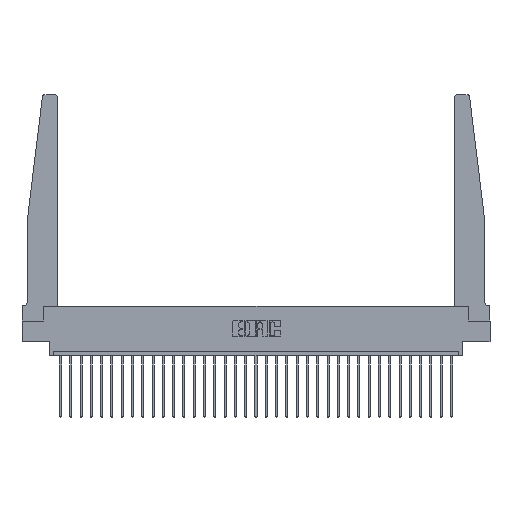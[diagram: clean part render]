
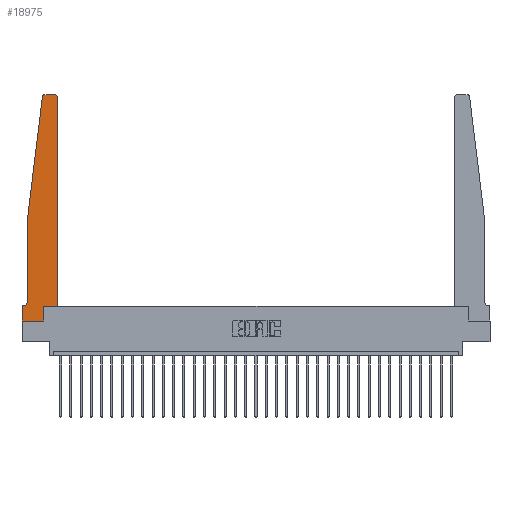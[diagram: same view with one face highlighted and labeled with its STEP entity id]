
A CAD part, top view. The second image highlights one B-rep face of the part: STEP entity #18975.
In plain terms, the highlighted planar face has unit normal (0, 0, 1).
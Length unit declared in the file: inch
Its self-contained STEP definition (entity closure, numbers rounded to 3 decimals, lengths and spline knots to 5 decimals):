
#232 = CARTESIAN_POINT ( 'NONE',  ( 0.065, 1.25, 0.37 ) ) ;
#612 = CARTESIAN_POINT ( 'NONE',  ( 0., 0.1875, 0.37 ) ) ;
#1583 = VERTEX_POINT ( 'NONE', #20414 ) ;
#1727 = DIRECTION ( 'NONE',  ( -1., 0., 0. ) ) ;
#2934 = VERTEX_POINT ( 'NONE', #27861 ) ;
#2939 = CARTESIAN_POINT ( 'NONE',  ( 0.27653, 2.72, 0.37 ) ) ;
#3016 = CARTESIAN_POINT ( 'NONE',  ( 0.065, 1.25, 0.37 ) ) ;
#3254 = AXIS2_PLACEMENT_3D ( 'NONE', #21858, #15500, #8918 ) ;
#3406 = VERTEX_POINT ( 'NONE', #26268 ) ;
#3511 = CARTESIAN_POINT ( 'NONE',  ( 0.395, 2.72, 0.37 ) ) ;
#3538 = CARTESIAN_POINT ( 'NONE',  ( 0.065, 1.25, 0.37 ) ) ;
#3747 = CARTESIAN_POINT ( 'NONE',  ( 0.065, 0.1875, 0.37 ) ) ;
#4135 = DIRECTION ( 'NONE',  ( 0., 0., -1. ) ) ;
#4173 = EDGE_CURVE ( 'NONE', #13566, #26030, #20560, .T. ) ;
#4426 = DIRECTION ( 'NONE',  ( 1., 0., 0. ) ) ;
#5262 = DIRECTION ( 'NONE',  ( 0., 1., 0. ) ) ;
#5278 = VERTEX_POINT ( 'NONE', #26256 ) ;
#5492 = CIRCLE ( 'NONE', #21734, 0.03 ) ;
#5751 = EDGE_CURVE ( 'NONE', #7166, #2934, #5492, .T. ) ;
#5842 = ORIENTED_EDGE ( 'NONE', *, *, #21548, .T. ) ;
#6036 = VERTEX_POINT ( 'NONE', #3538 ) ;
#6466 = CARTESIAN_POINT ( 'NONE',  ( 0.2605, 0.18, 0.37 ) ) ;
#6609 = ORIENTED_EDGE ( 'NONE', *, *, #5751, .T. ) ;
#6763 = EDGE_CURVE ( 'NONE', #5278, #23042, #8334, .T. ) ;
#7166 = VERTEX_POINT ( 'NONE', #9175 ) ;
#7581 = LINE ( 'NONE', #3747, #11492 ) ;
#7905 = CARTESIAN_POINT ( 'NONE',  ( 0.2605, 0., 0.37 ) ) ;
#8334 = CIRCLE ( 'NONE', #17591, 0.03 ) ;
#8335 = VECTOR ( 'NONE', #13988, 39.37008 ) ;
#8407 = EDGE_LOOP ( 'NONE', ( #16401, #24054, #27686, #21532, #26151, #25144, #13466, #16204, #27030, #24911, #5842, #6609 ) ) ;
#8863 = CARTESIAN_POINT ( 'NONE',  ( 0.24675, 2.72367, 0.37 ) ) ;
#8918 = DIRECTION ( 'NONE',  ( 1., 0., 0. ) ) ;
#9175 = CARTESIAN_POINT ( 'NONE',  ( 0.425, 2.72, 0.37 ) ) ;
#9806 = LINE ( 'NONE', #22741, #27277 ) ;
#9874 = DIRECTION ( 'NONE',  ( 0., 0., 1. ) ) ;
#10101 = LINE ( 'NONE', #3016, #8335 ) ;
#10420 = PLANE ( 'NONE',  #3254 ) ;
#10680 = CARTESIAN_POINT ( 'NONE',  ( 0.425, 0.18, 0.37 ) ) ;
#11492 = VECTOR ( 'NONE', #1727, 39.37008 ) ;
#11778 = CARTESIAN_POINT ( 'NONE',  ( 0., 0., 0.37 ) ) ;
#12371 = EDGE_CURVE ( 'NONE', #3406, #17073, #15193, .T. ) ;
#13014 = EDGE_CURVE ( 'NONE', #17073, #13566, #28671, .T. ) ;
#13466 = ORIENTED_EDGE ( 'NONE', *, *, #22333, .T. ) ;
#13566 = VERTEX_POINT ( 'NONE', #6466 ) ;
#13734 = EDGE_CURVE ( 'NONE', #23042, #6036, #17628, .T. ) ;
#13781 = DIRECTION ( 'NONE',  ( -0.122, -0.992, 0. ) ) ;
#13988 = DIRECTION ( 'NONE',  ( 0., -1., 0. ) ) ;
#14502 = VECTOR ( 'NONE', #15463, 39.37008 ) ;
#15193 = LINE ( 'NONE', #18093, #19811 ) ;
#15463 = DIRECTION ( 'NONE',  ( 1., 0., 0. ) ) ;
#15468 = VECTOR ( 'NONE', #20947, 39.37008 ) ;
#15500 = DIRECTION ( 'NONE',  ( 0., 0., 1. ) ) ;
#15824 = VECTOR ( 'NONE', #13781, 39.37008 ) ;
#15874 = CARTESIAN_POINT ( 'NONE',  ( 0.015, 0.2375, 0.37 ) ) ;
#16204 = ORIENTED_EDGE ( 'NONE', *, *, #12371, .T. ) ;
#16401 = ORIENTED_EDGE ( 'NONE', *, *, #26616, .T. ) ;
#16575 = EDGE_CURVE ( 'NONE', #6036, #1583, #10101, .T. ) ;
#17073 = VERTEX_POINT ( 'NONE', #7905 ) ;
#17575 = DIRECTION ( 'NONE',  ( 0., 1., 0. ) ) ;
#17591 = AXIS2_PLACEMENT_3D ( 'NONE', #2939, #18895, #23479 ) ;
#17628 = LINE ( 'NONE', #232, #15824 ) ;
#18093 = CARTESIAN_POINT ( 'NONE',  ( 0., 0., 0.37 ) ) ;
#18745 = VECTOR ( 'NONE', #22228, 39.37008 ) ;
#18895 = DIRECTION ( 'NONE',  ( 0., 0., 1. ) ) ;
#18975 = ADVANCED_FACE ( 'NONE', ( #24585 ), #10420, .T. ) ;
#19687 = CIRCLE ( 'NONE', #25252, 0.05 ) ;
#19811 = VECTOR ( 'NONE', #4426, 39.37008 ) ;
#20017 = VERTEX_POINT ( 'NONE', #612 ) ;
#20414 = CARTESIAN_POINT ( 'NONE',  ( 0.065, 0.2375, 0.37 ) ) ;
#20560 = LINE ( 'NONE', #10680, #14502 ) ;
#20813 = CARTESIAN_POINT ( 'NONE',  ( 0.015, 0.1875, 0.37 ) ) ;
#20947 = DIRECTION ( 'NONE',  ( 0., -1., 0. ) ) ;
#21141 = CARTESIAN_POINT ( 'NONE',  ( 0.2605, 0.18, 0.37 ) ) ;
#21532 = ORIENTED_EDGE ( 'NONE', *, *, #16575, .T. ) ;
#21548 = EDGE_CURVE ( 'NONE', #26030, #7166, #9806, .T. ) ;
#21734 = AXIS2_PLACEMENT_3D ( 'NONE', #3511, #9874, #28308 ) ;
#21858 = CARTESIAN_POINT ( 'NONE',  ( 0., 0.1875, 0.37 ) ) ;
#22228 = DIRECTION ( 'NONE',  ( -1., 0., 0. ) ) ;
#22292 = LINE ( 'NONE', #29004, #18745 ) ;
#22333 = EDGE_CURVE ( 'NONE', #20017, #3406, #28302, .T. ) ;
#22614 = VERTEX_POINT ( 'NONE', #20813 ) ;
#22631 = VECTOR ( 'NONE', #17575, 39.37008 ) ;
#22643 = DIRECTION ( 'NONE',  ( -1., 0., 0. ) ) ;
#22741 = CARTESIAN_POINT ( 'NONE',  ( 0.425, 0.18, 0.37 ) ) ;
#23042 = VERTEX_POINT ( 'NONE', #8863 ) ;
#23479 = DIRECTION ( 'NONE',  ( 1., 0., 0. ) ) ;
#24054 = ORIENTED_EDGE ( 'NONE', *, *, #6763, .T. ) ;
#24585 = FACE_OUTER_BOUND ( 'NONE', #8407, .T. ) ;
#24911 = ORIENTED_EDGE ( 'NONE', *, *, #4173, .T. ) ;
#25144 = ORIENTED_EDGE ( 'NONE', *, *, #28240, .T. ) ;
#25252 = AXIS2_PLACEMENT_3D ( 'NONE', #15874, #4135, #22643 ) ;
#26030 = VERTEX_POINT ( 'NONE', #27153 ) ;
#26151 = ORIENTED_EDGE ( 'NONE', *, *, #28417, .T. ) ;
#26256 = CARTESIAN_POINT ( 'NONE',  ( 0.27653, 2.75, 0.37 ) ) ;
#26268 = CARTESIAN_POINT ( 'NONE',  ( 0., 0., 0.37 ) ) ;
#26616 = EDGE_CURVE ( 'NONE', #2934, #5278, #22292, .T. ) ;
#27030 = ORIENTED_EDGE ( 'NONE', *, *, #13014, .T. ) ;
#27153 = CARTESIAN_POINT ( 'NONE',  ( 0.425, 0.18, 0.37 ) ) ;
#27277 = VECTOR ( 'NONE', #5262, 39.37008 ) ;
#27686 = ORIENTED_EDGE ( 'NONE', *, *, #13734, .T. ) ;
#27861 = CARTESIAN_POINT ( 'NONE',  ( 0.395, 2.75, 0.37 ) ) ;
#28240 = EDGE_CURVE ( 'NONE', #22614, #20017, #7581, .T. ) ;
#28302 = LINE ( 'NONE', #11778, #15468 ) ;
#28308 = DIRECTION ( 'NONE',  ( 1., 0., 0. ) ) ;
#28417 = EDGE_CURVE ( 'NONE', #1583, #22614, #19687, .T. ) ;
#28671 = LINE ( 'NONE', #21141, #22631 ) ;
#29004 = CARTESIAN_POINT ( 'NONE',  ( 0.25, 2.75, 0.37 ) ) ;
